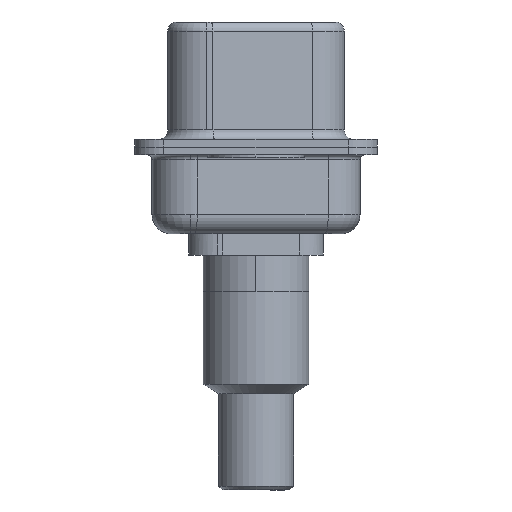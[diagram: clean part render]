
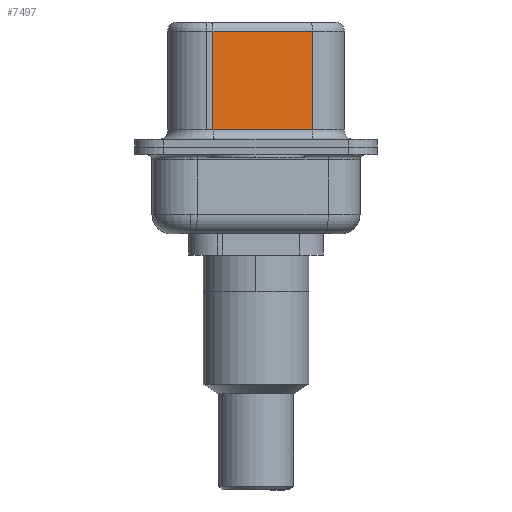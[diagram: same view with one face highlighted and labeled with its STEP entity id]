
A CAD part, left-side view. The second image highlights one B-rep face of the part: STEP entity #7497.
In plain terms, the highlighted planar face has unit normal (-0.985, -0.174, 0).
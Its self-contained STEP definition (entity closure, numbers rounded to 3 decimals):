
#190 = VERTEX_POINT ( 'NONE', #9300 ) ;
#365 = DIRECTION ( 'NONE',  ( 0.174, -0.985, 0. ) ) ;
#824 = ORIENTED_EDGE ( 'NONE', *, *, #10709, .T. ) ;
#1033 = DIRECTION ( 'NONE',  ( -0.174, 0.985, 0. ) ) ;
#1503 = VERTEX_POINT ( 'NONE', #7082 ) ;
#1604 = EDGE_CURVE ( 'NONE', #190, #7266, #10839, .T. ) ;
#1639 = DIRECTION ( 'NONE',  ( -0.174, 0.985, 0. ) ) ;
#1896 = CARTESIAN_POINT ( 'NONE',  ( 3.675, 2.233, 6.52 ) ) ;
#2675 = CARTESIAN_POINT ( 'NONE',  ( 4.585, -2.927, 6.52 ) ) ;
#2713 = VERTEX_POINT ( 'NONE', #16503 ) ;
#3203 = ORIENTED_EDGE ( 'NONE', *, *, #12976, .F. ) ;
#4111 = LINE ( 'NONE', #1896, #8412 ) ;
#4438 = ORIENTED_EDGE ( 'NONE', *, *, #10807, .T. ) ;
#5013 = VECTOR ( 'NONE', #1639, 1000. ) ;
#7082 = CARTESIAN_POINT ( 'NONE',  ( 4.585, -2.927, 6.02 ) ) ;
#7266 = VERTEX_POINT ( 'NONE', #13673 ) ;
#7497 = ADVANCED_FACE ( 'NONE', ( #8938 ), #15781, .F. ) ;
#8412 = VECTOR ( 'NONE', #9109, 1000. ) ;
#8913 = CARTESIAN_POINT ( 'NONE',  ( 4.585, -2.927, 6.02 ) ) ;
#8938 = FACE_OUTER_BOUND ( 'NONE', #18429, .T. ) ;
#9109 = DIRECTION ( 'NONE',  ( 0., 0., -1. ) ) ;
#9300 = CARTESIAN_POINT ( 'NONE',  ( 3.675, 2.233, 0.9 ) ) ;
#9728 = CARTESIAN_POINT ( 'NONE',  ( 4.585, -2.927, 0.9 ) ) ;
#10709 = EDGE_CURVE ( 'NONE', #1503, #2713, #13588, .T. ) ;
#10807 = EDGE_CURVE ( 'NONE', #2713, #190, #4111, .T. ) ;
#10839 = LINE ( 'NONE', #9728, #13779 ) ;
#10984 = ORIENTED_EDGE ( 'NONE', *, *, #1604, .T. ) ;
#11313 = CARTESIAN_POINT ( 'NONE',  ( 4.585, -2.927, 6.52 ) ) ;
#12976 = EDGE_CURVE ( 'NONE', #1503, #7266, #18506, .T. ) ;
#13588 = LINE ( 'NONE', #8913, #5013 ) ;
#13673 = CARTESIAN_POINT ( 'NONE',  ( 4.585, -2.927, 0.9 ) ) ;
#13779 = VECTOR ( 'NONE', #365, 1000. ) ;
#14636 = VECTOR ( 'NONE', #18578, 1000. ) ;
#15781 = PLANE ( 'NONE',  #15983 ) ;
#15983 = AXIS2_PLACEMENT_3D ( 'NONE', #11313, #18486, #1033 ) ;
#16503 = CARTESIAN_POINT ( 'NONE',  ( 3.675, 2.233, 6.02 ) ) ;
#18429 = EDGE_LOOP ( 'NONE', ( #3203, #824, #4438, #10984 ) ) ;
#18486 = DIRECTION ( 'NONE',  ( 0.985, 0.174, 0. ) ) ;
#18506 = LINE ( 'NONE', #2675, #14636 ) ;
#18578 = DIRECTION ( 'NONE',  ( 0., 0., -1. ) ) ;
